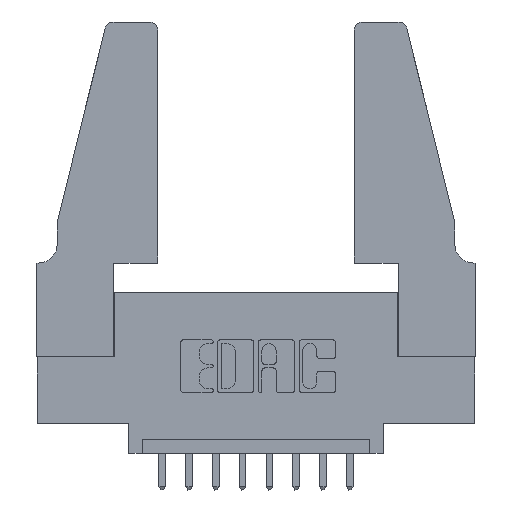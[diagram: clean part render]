
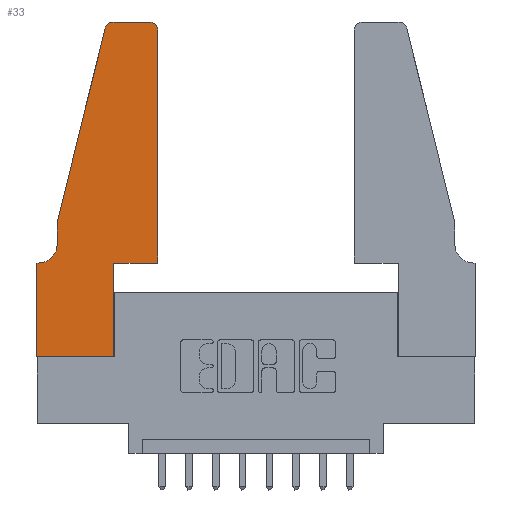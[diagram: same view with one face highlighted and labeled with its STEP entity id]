
A CAD part, top view. The second image highlights one B-rep face of the part: STEP entity #33.
In plain terms, the highlighted planar face has unit normal (0, 0, 1).
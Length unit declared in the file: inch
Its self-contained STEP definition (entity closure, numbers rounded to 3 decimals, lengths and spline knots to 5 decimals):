
#33 = ADVANCED_FACE ( 'NONE', ( #9271 ), #1109, .T. ) ;
#222 = LINE ( 'NONE', #3610, #11916 ) ;
#227 = EDGE_CURVE ( 'NONE', #1021, #12560, #222, .T. ) ;
#309 = LINE ( 'NONE', #7969, #7630 ) ;
#351 = CIRCLE ( 'NONE', #8754, 0.03 ) ;
#452 = DIRECTION ( 'NONE',  ( 0., 0., 1. ) ) ;
#1016 = ORIENTED_EDGE ( 'NONE', *, *, #4951, .T. ) ;
#1021 = VERTEX_POINT ( 'NONE', #7850 ) ;
#1024 = CARTESIAN_POINT ( 'NONE',  ( 0.4205, 1.22, 0.37 ) ) ;
#1109 = PLANE ( 'NONE',  #1813 ) ;
#1164 = ORIENTED_EDGE ( 'NONE', *, *, #9197, .T. ) ;
#1319 = ORIENTED_EDGE ( 'NONE', *, *, #7568, .T. ) ;
#1553 = ORIENTED_EDGE ( 'NONE', *, *, #7180, .T. ) ;
#1738 = LINE ( 'NONE', #5149, #12467 ) ;
#1749 = VERTEX_POINT ( 'NONE', #1807 ) ;
#1807 = CARTESIAN_POINT ( 'NONE',  ( 0.2865, 0., 0.37 ) ) ;
#1813 = AXIS2_PLACEMENT_3D ( 'NONE', #8113, #12136, #2145 ) ;
#1985 = CIRCLE ( 'NONE', #6915, 0.03 ) ;
#1990 = VERTEX_POINT ( 'NONE', #5337 ) ;
#2048 = CARTESIAN_POINT ( 'NONE',  ( 0.4505, 1.22, 0.37 ) ) ;
#2063 = DIRECTION ( 'NONE',  ( 0., 0., 1. ) ) ;
#2145 = DIRECTION ( 'NONE',  ( 1., 0., 0. ) ) ;
#2516 = LINE ( 'NONE', #4058, #12922 ) ;
#2657 = DIRECTION ( 'NONE',  ( 0., 1., 0. ) ) ;
#2757 = CARTESIAN_POINT ( 'NONE',  ( 0.2605, 1.25, 0.37 ) ) ;
#2766 = ORIENTED_EDGE ( 'NONE', *, *, #9835, .T. ) ;
#3170 = EDGE_CURVE ( 'NONE', #9081, #10926, #5773, .T. ) ;
#3231 = EDGE_LOOP ( 'NONE', ( #8016, #1553, #1164, #5101, #1016, #11545, #9263, #1319, #4998, #2766, #12741, #8089 ) ) ;
#3241 = CIRCLE ( 'NONE', #10752, 0.07 ) ;
#3610 = CARTESIAN_POINT ( 'NONE',  ( 0.4505, 0.35, 0.37 ) ) ;
#3698 = CARTESIAN_POINT ( 'NONE',  ( 0.284, 1.25, 0.37 ) ) ;
#4058 = CARTESIAN_POINT ( 'NONE',  ( 0.0755, 0.5, 0.37 ) ) ;
#4216 = VECTOR ( 'NONE', #7818, 39.37008 ) ;
#4267 = DIRECTION ( 'NONE',  ( 0., -1., 0. ) ) ;
#4434 = CARTESIAN_POINT ( 'NONE',  ( 0., 0., 0.37 ) ) ;
#4721 = CARTESIAN_POINT ( 'NONE',  ( 0., 0., 0.37 ) ) ;
#4841 = DIRECTION ( 'NONE',  ( 0., 0., -1. ) ) ;
#4908 = CARTESIAN_POINT ( 'NONE',  ( 0.2865, 0.35, 0.37 ) ) ;
#4951 = EDGE_CURVE ( 'NONE', #10926, #6736, #3241, .T. ) ;
#4998 = ORIENTED_EDGE ( 'NONE', *, *, #9086, .T. ) ;
#5101 = ORIENTED_EDGE ( 'NONE', *, *, #3170, .T. ) ;
#5108 = CARTESIAN_POINT ( 'NONE',  ( 0., 0., 0.37 ) ) ;
#5146 = CARTESIAN_POINT ( 'NONE',  ( 0.2865, 0.35, 0.37 ) ) ;
#5149 = CARTESIAN_POINT ( 'NONE',  ( 0.4505, 0.35, 0.37 ) ) ;
#5337 = CARTESIAN_POINT ( 'NONE',  ( 0.4205, 1.25, 0.37 ) ) ;
#5534 = VERTEX_POINT ( 'NONE', #5108 ) ;
#5665 = DIRECTION ( 'NONE',  ( 0., -1., 0. ) ) ;
#5747 = DIRECTION ( 'NONE',  ( -1., 0., 0. ) ) ;
#5773 = LINE ( 'NONE', #7825, #10889 ) ;
#5845 = EDGE_CURVE ( 'NONE', #12560, #1990, #1985, .T. ) ;
#6586 = VECTOR ( 'NONE', #11516, 39.37008 ) ;
#6634 = CARTESIAN_POINT ( 'NONE',  ( 0.0755, 0.5, 0.37 ) ) ;
#6736 = VERTEX_POINT ( 'NONE', #8782 ) ;
#6915 = AXIS2_PLACEMENT_3D ( 'NONE', #1024, #2063, #9220 ) ;
#7180 = EDGE_CURVE ( 'NONE', #11351, #8840, #351, .T. ) ;
#7418 = DIRECTION ( 'NONE',  ( 1., 0., 0. ) ) ;
#7452 = LINE ( 'NONE', #2757, #4216 ) ;
#7568 = EDGE_CURVE ( 'NONE', #5534, #1749, #9230, .T. ) ;
#7630 = VECTOR ( 'NONE', #12896, 39.37008 ) ;
#7634 = DIRECTION ( 'NONE',  ( 0., 1., 0. ) ) ;
#7818 = DIRECTION ( 'NONE',  ( -1., 0., 0. ) ) ;
#7825 = CARTESIAN_POINT ( 'NONE',  ( 0.0755, 0.5, 0.37 ) ) ;
#7850 = CARTESIAN_POINT ( 'NONE',  ( 0.4505, 0.35, 0.37 ) ) ;
#7946 = LINE ( 'NONE', #4721, #9821 ) ;
#7969 = CARTESIAN_POINT ( 'NONE',  ( 0.0755, 0.35, 0.37 ) ) ;
#8016 = ORIENTED_EDGE ( 'NONE', *, *, #9577, .T. ) ;
#8089 = ORIENTED_EDGE ( 'NONE', *, *, #5845, .T. ) ;
#8113 = CARTESIAN_POINT ( 'NONE',  ( 0., 0.35, 0.37 ) ) ;
#8754 = AXIS2_PLACEMENT_3D ( 'NONE', #12355, #452, #7418 ) ;
#8782 = CARTESIAN_POINT ( 'NONE',  ( 0.0055, 0.35, 0.37 ) ) ;
#8840 = VERTEX_POINT ( 'NONE', #11269 ) ;
#9081 = VERTEX_POINT ( 'NONE', #6634 ) ;
#9086 = EDGE_CURVE ( 'NONE', #1749, #11915, #12000, .T. ) ;
#9149 = EDGE_CURVE ( 'NONE', #6736, #11780, #309, .T. ) ;
#9197 = EDGE_CURVE ( 'NONE', #8840, #9081, #2516, .T. ) ;
#9220 = DIRECTION ( 'NONE',  ( 1., 0., 0. ) ) ;
#9230 = LINE ( 'NONE', #4434, #6586 ) ;
#9263 = ORIENTED_EDGE ( 'NONE', *, *, #11703, .T. ) ;
#9271 = FACE_OUTER_BOUND ( 'NONE', #3231, .T. ) ;
#9577 = EDGE_CURVE ( 'NONE', #1990, #11351, #7452, .T. ) ;
#9658 = VECTOR ( 'NONE', #7634, 39.37008 ) ;
#9821 = VECTOR ( 'NONE', #5665, 39.37008 ) ;
#9835 = EDGE_CURVE ( 'NONE', #11915, #1021, #1738, .T. ) ;
#10010 = DIRECTION ( 'NONE',  ( -0.239, -0.971, 0. ) ) ;
#10034 = CARTESIAN_POINT ( 'NONE',  ( 0.0755, 0.42, 0.37 ) ) ;
#10752 = AXIS2_PLACEMENT_3D ( 'NONE', #10786, #4841, #5747 ) ;
#10786 = CARTESIAN_POINT ( 'NONE',  ( 0.0055, 0.42, 0.37 ) ) ;
#10889 = VECTOR ( 'NONE', #4267, 39.37008 ) ;
#10926 = VERTEX_POINT ( 'NONE', #10034 ) ;
#11003 = DIRECTION ( 'NONE',  ( 1., 0., 0. ) ) ;
#11269 = CARTESIAN_POINT ( 'NONE',  ( 0.25487, 1.22718, 0.37 ) ) ;
#11351 = VERTEX_POINT ( 'NONE', #3698 ) ;
#11516 = DIRECTION ( 'NONE',  ( 1., 0., 0. ) ) ;
#11545 = ORIENTED_EDGE ( 'NONE', *, *, #9149, .T. ) ;
#11703 = EDGE_CURVE ( 'NONE', #11780, #5534, #7946, .T. ) ;
#11780 = VERTEX_POINT ( 'NONE', #11891 ) ;
#11891 = CARTESIAN_POINT ( 'NONE',  ( 0., 0.35, 0.37 ) ) ;
#11915 = VERTEX_POINT ( 'NONE', #5146 ) ;
#11916 = VECTOR ( 'NONE', #2657, 39.37008 ) ;
#12000 = LINE ( 'NONE', #4908, #9658 ) ;
#12136 = DIRECTION ( 'NONE',  ( 0., 0., 1. ) ) ;
#12355 = CARTESIAN_POINT ( 'NONE',  ( 0.284, 1.22, 0.37 ) ) ;
#12467 = VECTOR ( 'NONE', #11003, 39.37008 ) ;
#12560 = VERTEX_POINT ( 'NONE', #2048 ) ;
#12741 = ORIENTED_EDGE ( 'NONE', *, *, #227, .T. ) ;
#12896 = DIRECTION ( 'NONE',  ( -1., 0., 0. ) ) ;
#12922 = VECTOR ( 'NONE', #10010, 39.37008 ) ;
